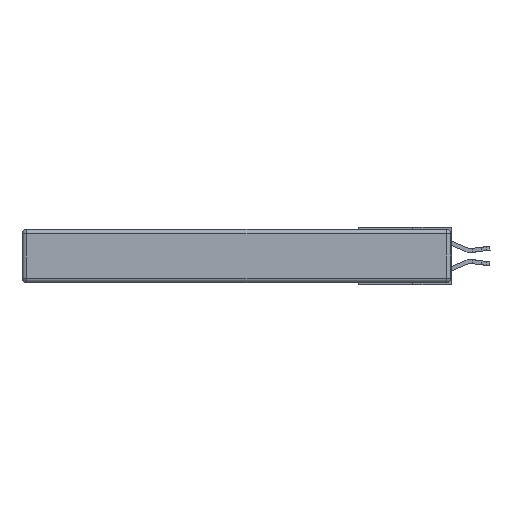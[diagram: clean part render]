
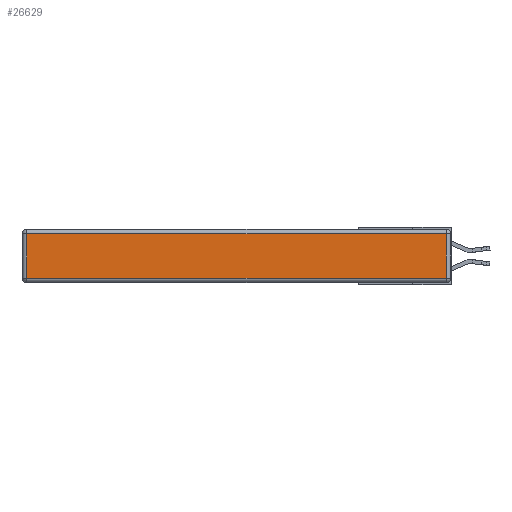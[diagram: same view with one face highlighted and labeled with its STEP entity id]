
A CAD part, left-side view. The second image highlights one B-rep face of the part: STEP entity #26629.
In plain terms, the highlighted planar face has unit normal (-1, 0, 0).
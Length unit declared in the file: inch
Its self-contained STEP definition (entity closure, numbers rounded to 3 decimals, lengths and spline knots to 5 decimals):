
#600 = VERTEX_POINT ( 'NONE', #19121 ) ;
#608 = PLANE ( 'NONE',  #8023 ) ;
#1862 = CARTESIAN_POINT ( 'NONE',  ( 0., 2.75, -0.03 ) ) ;
#3513 = VECTOR ( 'NONE', #10760, 39.37008 ) ;
#3989 = ORIENTED_EDGE ( 'NONE', *, *, #20960, .T. ) ;
#4027 = CARTESIAN_POINT ( 'NONE',  ( 0., 2.72, -0.343 ) ) ;
#4805 = LINE ( 'NONE', #20983, #3513 ) ;
#5610 = DIRECTION ( 'NONE',  ( -1., 0., 0. ) ) ;
#5733 = VERTEX_POINT ( 'NONE', #23061 ) ;
#6036 = EDGE_LOOP ( 'NONE', ( #13984, #23662, #3989, #13802 ) ) ;
#6293 = VECTOR ( 'NONE', #21819, 39.37008 ) ;
#6968 = EDGE_CURVE ( 'NONE', #600, #21081, #25772, .T. ) ;
#7387 = DIRECTION ( 'NONE',  ( 0., 0., 1. ) ) ;
#7677 = CARTESIAN_POINT ( 'NONE',  ( 0., 0., -0.343 ) ) ;
#8023 = AXIS2_PLACEMENT_3D ( 'NONE', #7677, #5610, #24053 ) ;
#8218 = CARTESIAN_POINT ( 'NONE',  ( 0., 0.03, -0.03 ) ) ;
#8783 = VECTOR ( 'NONE', #7387, 39.37008 ) ;
#9024 = LINE ( 'NONE', #4027, #13507 ) ;
#10760 = DIRECTION ( 'NONE',  ( 0., -1., 0. ) ) ;
#12731 = VERTEX_POINT ( 'NONE', #16800 ) ;
#13507 = VECTOR ( 'NONE', #24380, 39.37008 ) ;
#13802 = ORIENTED_EDGE ( 'NONE', *, *, #14164, .T. ) ;
#13984 = ORIENTED_EDGE ( 'NONE', *, *, #14076, .T. ) ;
#14076 = EDGE_CURVE ( 'NONE', #12731, #600, #4805, .T. ) ;
#14164 = EDGE_CURVE ( 'NONE', #5733, #12731, #9024, .T. ) ;
#14388 = FACE_OUTER_BOUND ( 'NONE', #6036, .T. ) ;
#16800 = CARTESIAN_POINT ( 'NONE',  ( 0., 2.72, -0.313 ) ) ;
#18508 = LINE ( 'NONE', #1862, #6293 ) ;
#19121 = CARTESIAN_POINT ( 'NONE',  ( 0., 0.03, -0.313 ) ) ;
#20960 = EDGE_CURVE ( 'NONE', #21081, #5733, #18508, .T. ) ;
#20983 = CARTESIAN_POINT ( 'NONE',  ( 0., 0., -0.313 ) ) ;
#21081 = VERTEX_POINT ( 'NONE', #8218 ) ;
#21819 = DIRECTION ( 'NONE',  ( 0., 1., 0. ) ) ;
#23061 = CARTESIAN_POINT ( 'NONE',  ( 0., 2.72, -0.03 ) ) ;
#23596 = CARTESIAN_POINT ( 'NONE',  ( 0., 0.03, -0.343 ) ) ;
#23662 = ORIENTED_EDGE ( 'NONE', *, *, #6968, .T. ) ;
#24053 = DIRECTION ( 'NONE',  ( 0., 0., 1. ) ) ;
#24380 = DIRECTION ( 'NONE',  ( 0., 0., -1. ) ) ;
#25772 = LINE ( 'NONE', #23596, #8783 ) ;
#26629 = ADVANCED_FACE ( 'NONE', ( #14388 ), #608, .T. ) ;
